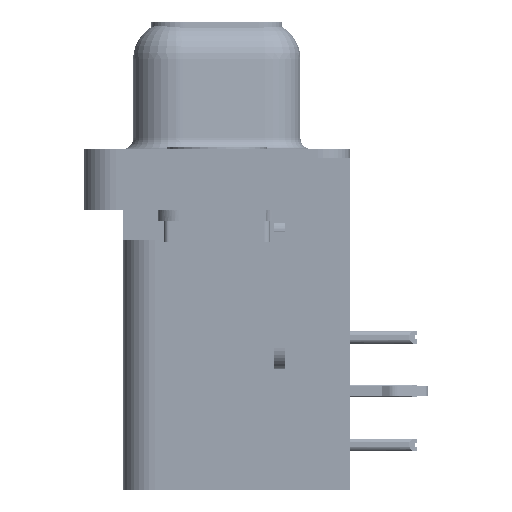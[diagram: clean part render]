
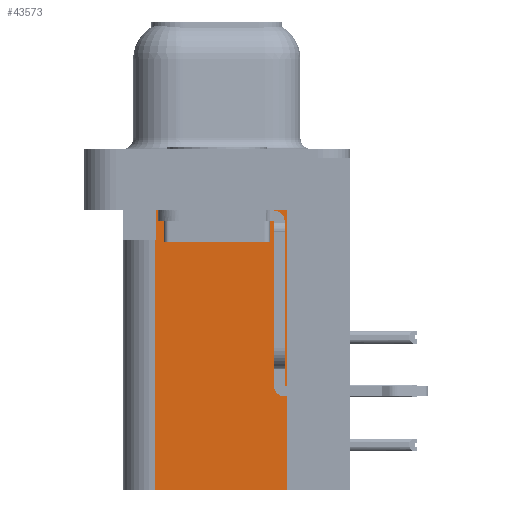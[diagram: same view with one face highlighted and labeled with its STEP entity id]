
A CAD part, left-side view. The second image highlights one B-rep face of the part: STEP entity #43573.
In plain terms, the highlighted planar face has unit normal (-1, 0, 0).
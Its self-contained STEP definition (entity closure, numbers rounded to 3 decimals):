
#1766 = VECTOR ( 'NONE', #26359, 1000. ) ;
#2370 = CARTESIAN_POINT ( 'NONE',  ( 3.79, 2.925, -15.7 ) ) ;
#2810 = LINE ( 'NONE', #32842, #35807 ) ;
#3709 = CARTESIAN_POINT ( 'NONE',  ( 3.79, 0., -3.9 ) ) ;
#5118 = CARTESIAN_POINT ( 'NONE',  ( 3.79, 2.895, -2.5 ) ) ;
#5132 = CARTESIAN_POINT ( 'NONE',  ( 3.79, 2.895, -3.9 ) ) ;
#5473 = CARTESIAN_POINT ( 'NONE',  ( 3.79, 2.925, -15.7 ) ) ;
#5896 = VERTEX_POINT ( 'NONE', #25247 ) ;
#6127 = AXIS2_PLACEMENT_3D ( 'NONE', #19643, #47081, #23686 ) ;
#6164 = CARTESIAN_POINT ( 'NONE',  ( 3.79, -3.295, -15.7 ) ) ;
#6221 = ORIENTED_EDGE ( 'NONE', *, *, #48125, .T. ) ;
#7540 = PLANE ( 'NONE',  #6127 ) ;
#7962 = DIRECTION ( 'NONE',  ( 0., 1., 0. ) ) ;
#8981 = DIRECTION ( 'NONE',  ( 0., 1., 0. ) ) ;
#9585 = EDGE_CURVE ( 'NONE', #14159, #46625, #2810, .T. ) ;
#10221 = EDGE_CURVE ( 'NONE', #38352, #14159, #42470, .T. ) ;
#12425 = ORIENTED_EDGE ( 'NONE', *, *, #9585, .T. ) ;
#12665 = ORIENTED_EDGE ( 'NONE', *, *, #10221, .T. ) ;
#14159 = VERTEX_POINT ( 'NONE', #43636 ) ;
#14868 = FACE_OUTER_BOUND ( 'NONE', #26479, .T. ) ;
#15417 = LINE ( 'NONE', #3709, #35223 ) ;
#16723 = EDGE_CURVE ( 'NONE', #46625, #5896, #29962, .T. ) ;
#18088 = DIRECTION ( 'NONE',  ( 0., 1., 0. ) ) ;
#18449 = ORIENTED_EDGE ( 'NONE', *, *, #31285, .F. ) ;
#19482 = VECTOR ( 'NONE', #48682, 1000. ) ;
#19643 = CARTESIAN_POINT ( 'NONE',  ( 3.79, -3.295, -15.7 ) ) ;
#23686 = DIRECTION ( 'NONE',  ( 0., 0., -1. ) ) ;
#25247 = CARTESIAN_POINT ( 'NONE',  ( 3.79, 2.895, -3.9 ) ) ;
#25721 = DIRECTION ( 'NONE',  ( 0., 0., 1. ) ) ;
#26359 = DIRECTION ( 'NONE',  ( 0., 0., 1. ) ) ;
#26479 = EDGE_LOOP ( 'NONE', ( #12425, #42324, #6221, #18449, #32741, #12665 ) ) ;
#29962 = LINE ( 'NONE', #5132, #19482 ) ;
#31285 = EDGE_CURVE ( 'NONE', #46668, #37224, #42760, .T. ) ;
#32093 = VECTOR ( 'NONE', #25721, 1000. ) ;
#32741 = ORIENTED_EDGE ( 'NONE', *, *, #46777, .F. ) ;
#32806 = VECTOR ( 'NONE', #18088, 1000. ) ;
#32842 = CARTESIAN_POINT ( 'NONE',  ( 3.79, -3.295, -2.5 ) ) ;
#35223 = VECTOR ( 'NONE', #7962, 1000. ) ;
#35807 = VECTOR ( 'NONE', #8981, 1000. ) ;
#37179 = CARTESIAN_POINT ( 'NONE',  ( 3.79, -3.295, -15.7 ) ) ;
#37224 = VERTEX_POINT ( 'NONE', #49601 ) ;
#38352 = VERTEX_POINT ( 'NONE', #37179 ) ;
#42324 = ORIENTED_EDGE ( 'NONE', *, *, #16723, .T. ) ;
#42470 = LINE ( 'NONE', #45174, #32093 ) ;
#42760 = LINE ( 'NONE', #2370, #1766 ) ;
#43573 = ADVANCED_FACE ( 'NONE', ( #14868 ), #7540, .F. ) ;
#43636 = CARTESIAN_POINT ( 'NONE',  ( 3.79, -3.295, -2.5 ) ) ;
#45174 = CARTESIAN_POINT ( 'NONE',  ( 3.79, -3.295, -15.7 ) ) ;
#45578 = LINE ( 'NONE', #6164, #32806 ) ;
#46625 = VERTEX_POINT ( 'NONE', #5118 ) ;
#46668 = VERTEX_POINT ( 'NONE', #5473 ) ;
#46777 = EDGE_CURVE ( 'NONE', #38352, #46668, #45578, .T. ) ;
#47081 = DIRECTION ( 'NONE',  ( 1., 0., 0. ) ) ;
#48125 = EDGE_CURVE ( 'NONE', #5896, #37224, #15417, .T. ) ;
#48682 = DIRECTION ( 'NONE',  ( 0., 0., -1. ) ) ;
#49601 = CARTESIAN_POINT ( 'NONE',  ( 3.79, 2.925, -3.9 ) ) ;
